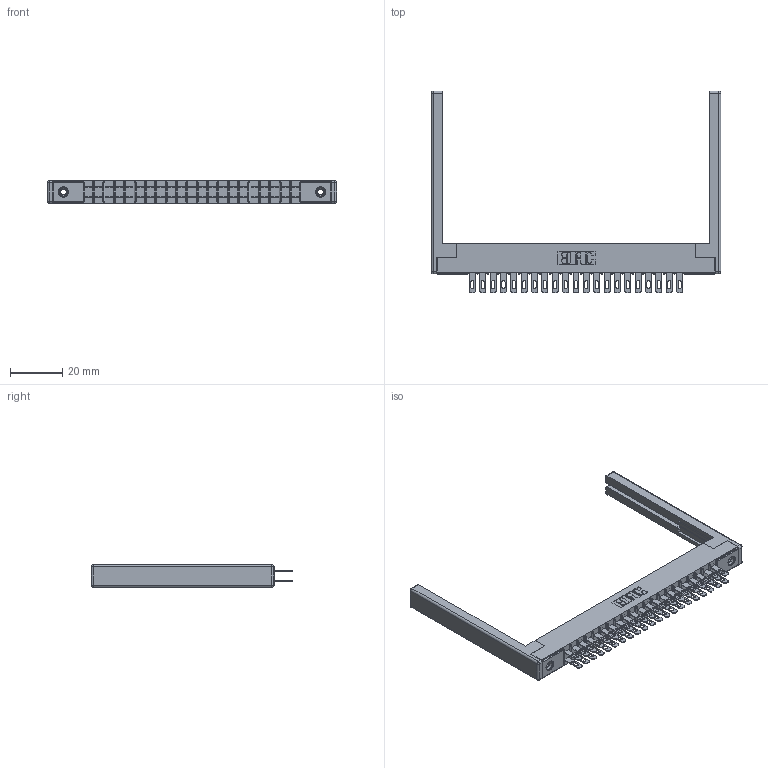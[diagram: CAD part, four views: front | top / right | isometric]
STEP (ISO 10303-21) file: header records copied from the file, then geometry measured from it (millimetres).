
FILE_DESCRIPTION (( 'STEP AP203' ), '1' );
FILE_NAME ('355-042-500-568.STEP', '2019-09-11T13:35:13', ( '' ), ( '' ), 'SwSTEP 2.0', 'SolidWorks 2016', '' );
FILE_SCHEMA (( 'CONFIG_CONTROL_DESIGN' ));
Length unit declared in the file: inch
Products named in the file (5): 345-250-001_345-250-001-102; 305-290-001_500; 305 Part_.156 Dia; 355-042-500-568; 307-220-068
Assembly tree (47 placements, depth 2):
  355-042-500-568
    305 Part_.156 Dia
    305-290-001_500  x42
    345-250-001_345-250-001-102  x2
    307-220-068  x2
Bounding box: 110.64 x 77.14 x 8.71 mm (x, y, z)
Volume: 11349.6 mm3; surface area: 18165.6 mm2
Topology: 47 solids, 47 shells, 2370 faces, 6733 edges, 4354 vertices
Faces by surface type: plane 1332, cylinder 930, sphere 92, cone 12, torus 4
Entity records: 28075 total; most frequent: CARTESIAN_POINT 4618, ORIENTED_EDGE 4572, DIRECTION 4506, EDGE_CURVE 2286, VECTOR 1814, LINE 1814, VERTEX_POINT 1458, AXIS2_PLACEMENT_3D 1346
